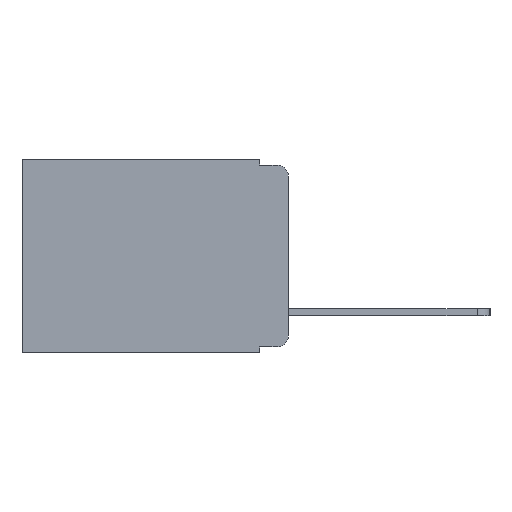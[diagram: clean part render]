
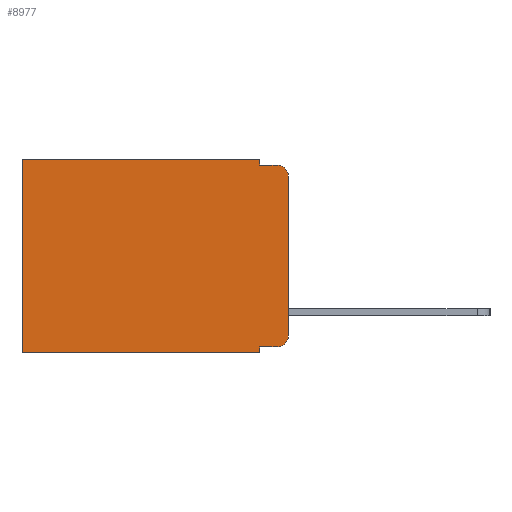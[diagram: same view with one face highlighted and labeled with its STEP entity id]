
A CAD part, left-side view. The second image highlights one B-rep face of the part: STEP entity #8977.
In plain terms, the highlighted planar face has unit normal (-1, 0, 0).
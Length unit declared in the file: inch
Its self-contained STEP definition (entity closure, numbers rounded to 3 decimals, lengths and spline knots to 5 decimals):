
#222 = VECTOR ( 'NONE', #14459, 39.37008 ) ;
#367 = CARTESIAN_POINT ( 'NONE',  ( 0.298, 0., 0. ) ) ;
#593 = CARTESIAN_POINT ( 'NONE',  ( 0.298, 0., 0. ) ) ;
#698 = CIRCLE ( 'NONE', #1022, 0.02 ) ;
#722 = VECTOR ( 'NONE', #9924, 39.37008 ) ;
#758 = AXIS2_PLACEMENT_3D ( 'NONE', #14933, #14852, #14511 ) ;
#855 = LINE ( 'NONE', #23486, #19789 ) ;
#1022 = AXIS2_PLACEMENT_3D ( 'NONE', #8545, #21256, #10366 ) ;
#1817 = CARTESIAN_POINT ( 'NONE',  ( 0.298, 0.051, -0.333 ) ) ;
#3137 = EDGE_CURVE ( 'NONE', #3982, #8626, #17443, .T. ) ;
#3230 = VERTEX_POINT ( 'NONE', #23293 ) ;
#3459 = DIRECTION ( 'NONE',  ( 0., 1., 0. ) ) ;
#3982 = VERTEX_POINT ( 'NONE', #1817 ) ;
#4323 = EDGE_CURVE ( 'NONE', #19435, #9033, #10548, .T. ) ;
#4376 = DIRECTION ( 'NONE',  ( 0., 0., -1. ) ) ;
#5673 = EDGE_LOOP ( 'NONE', ( #6289, #20471, #17805, #6717, #12734, #8162, #19860, #14484, #6816, #5957 ) ) ;
#5852 = EDGE_CURVE ( 'NONE', #19912, #16352, #6726, .T. ) ;
#5957 = ORIENTED_EDGE ( 'NONE', *, *, #11367, .T. ) ;
#6002 = DIRECTION ( 'NONE',  ( 0., 0., -1. ) ) ;
#6033 = CARTESIAN_POINT ( 'NONE',  ( 0.298, 0., -0.313 ) ) ;
#6289 = ORIENTED_EDGE ( 'NONE', *, *, #11917, .F. ) ;
#6717 = ORIENTED_EDGE ( 'NONE', *, *, #11127, .F. ) ;
#6726 = CIRCLE ( 'NONE', #758, 0.02 ) ;
#6816 = ORIENTED_EDGE ( 'NONE', *, *, #17508, .T. ) ;
#6835 = VERTEX_POINT ( 'NONE', #6033 ) ;
#7468 = DIRECTION ( 'NONE',  ( 0., 0., -1. ) ) ;
#7972 = PLANE ( 'NONE',  #19878 ) ;
#8162 = ORIENTED_EDGE ( 'NONE', *, *, #10484, .T. ) ;
#8545 = CARTESIAN_POINT ( 'NONE',  ( 0.298, 0.02, -0.313 ) ) ;
#8626 = VERTEX_POINT ( 'NONE', #17763 ) ;
#8970 = VECTOR ( 'NONE', #7468, 39.37008 ) ;
#8977 = ADVANCED_FACE ( 'NONE', ( #12212 ), #7972, .F. ) ;
#9033 = VERTEX_POINT ( 'NONE', #19022 ) ;
#9228 = VECTOR ( 'NONE', #18017, 39.37008 ) ;
#9924 = DIRECTION ( 'NONE',  ( 0., 1., 0. ) ) ;
#10026 = CARTESIAN_POINT ( 'NONE',  ( 0.298, 0.051, -0.01 ) ) ;
#10107 = DIRECTION ( 'NONE',  ( 0., 0., -1. ) ) ;
#10366 = DIRECTION ( 'NONE',  ( 0., 0., -1. ) ) ;
#10484 = EDGE_CURVE ( 'NONE', #9033, #13418, #22672, .T. ) ;
#10548 = LINE ( 'NONE', #367, #722 ) ;
#10886 = CARTESIAN_POINT ( 'NONE',  ( 0.298, 0.051, -0.01 ) ) ;
#11127 = EDGE_CURVE ( 'NONE', #19435, #21316, #13842, .T. ) ;
#11367 = EDGE_CURVE ( 'NONE', #3230, #6835, #698, .T. ) ;
#11909 = VECTOR ( 'NONE', #10107, 39.37008 ) ;
#11917 = EDGE_CURVE ( 'NONE', #19912, #6835, #16768, .T. ) ;
#12212 = FACE_OUTER_BOUND ( 'NONE', #5673, .T. ) ;
#12355 = LINE ( 'NONE', #10886, #9228 ) ;
#12525 = CARTESIAN_POINT ( 'NONE',  ( 0.298, 0.051, -0.333 ) ) ;
#12734 = ORIENTED_EDGE ( 'NONE', *, *, #4323, .T. ) ;
#12745 = CARTESIAN_POINT ( 'NONE',  ( 0.298, 0.02, -0.01 ) ) ;
#13418 = VERTEX_POINT ( 'NONE', #13983 ) ;
#13842 = LINE ( 'NONE', #21917, #8970 ) ;
#13983 = CARTESIAN_POINT ( 'NONE',  ( 0.298, 0.473, -0.343 ) ) ;
#14459 = DIRECTION ( 'NONE',  ( 0., -1., 0. ) ) ;
#14484 = ORIENTED_EDGE ( 'NONE', *, *, #3137, .F. ) ;
#14511 = DIRECTION ( 'NONE',  ( 0., 0., -1. ) ) ;
#14834 = EDGE_CURVE ( 'NONE', #21316, #16352, #12355, .T. ) ;
#14852 = DIRECTION ( 'NONE',  ( -1., 0., 0. ) ) ;
#14901 = LINE ( 'NONE', #12525, #222 ) ;
#14933 = CARTESIAN_POINT ( 'NONE',  ( 0.298, 0.02, -0.03 ) ) ;
#15312 = DIRECTION ( 'NONE',  ( 1., 0., 0. ) ) ;
#15559 = CARTESIAN_POINT ( 'NONE',  ( 0.298, 0.051, 0. ) ) ;
#16352 = VERTEX_POINT ( 'NONE', #12745 ) ;
#16469 = CARTESIAN_POINT ( 'NONE',  ( 0.298, 0.473, 0. ) ) ;
#16768 = LINE ( 'NONE', #20994, #11909 ) ;
#17443 = LINE ( 'NONE', #23348, #21121 ) ;
#17508 = EDGE_CURVE ( 'NONE', #3982, #3230, #14901, .T. ) ;
#17763 = CARTESIAN_POINT ( 'NONE',  ( 0.298, 0.051, -0.343 ) ) ;
#17805 = ORIENTED_EDGE ( 'NONE', *, *, #14834, .F. ) ;
#18017 = DIRECTION ( 'NONE',  ( 0., -1., 0. ) ) ;
#18282 = DIRECTION ( 'NONE',  ( 0., 0., -1. ) ) ;
#18382 = VECTOR ( 'NONE', #18282, 39.37008 ) ;
#18744 = CARTESIAN_POINT ( 'NONE',  ( 0.298, 0., -0.03 ) ) ;
#19022 = CARTESIAN_POINT ( 'NONE',  ( 0.298, 0.473, 0. ) ) ;
#19435 = VERTEX_POINT ( 'NONE', #15559 ) ;
#19789 = VECTOR ( 'NONE', #3459, 39.37008 ) ;
#19860 = ORIENTED_EDGE ( 'NONE', *, *, #22654, .F. ) ;
#19878 = AXIS2_PLACEMENT_3D ( 'NONE', #593, #15312, #4376 ) ;
#19912 = VERTEX_POINT ( 'NONE', #18744 ) ;
#20471 = ORIENTED_EDGE ( 'NONE', *, *, #5852, .T. ) ;
#20994 = CARTESIAN_POINT ( 'NONE',  ( 0.298, 0., 0. ) ) ;
#21121 = VECTOR ( 'NONE', #6002, 39.37008 ) ;
#21256 = DIRECTION ( 'NONE',  ( -1., 0., 0. ) ) ;
#21316 = VERTEX_POINT ( 'NONE', #10026 ) ;
#21917 = CARTESIAN_POINT ( 'NONE',  ( 0.298, 0.051, 0. ) ) ;
#22654 = EDGE_CURVE ( 'NONE', #8626, #13418, #855, .T. ) ;
#22672 = LINE ( 'NONE', #16469, #18382 ) ;
#23293 = CARTESIAN_POINT ( 'NONE',  ( 0.298, 0.02, -0.333 ) ) ;
#23348 = CARTESIAN_POINT ( 'NONE',  ( 0.298, 0.051, 0. ) ) ;
#23486 = CARTESIAN_POINT ( 'NONE',  ( 0.298, 0., -0.343 ) ) ;
